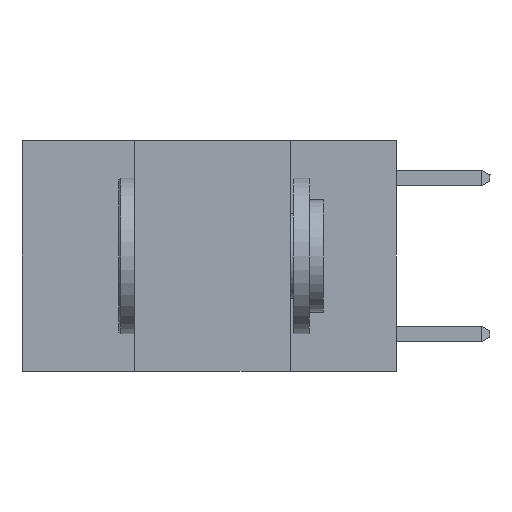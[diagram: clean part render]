
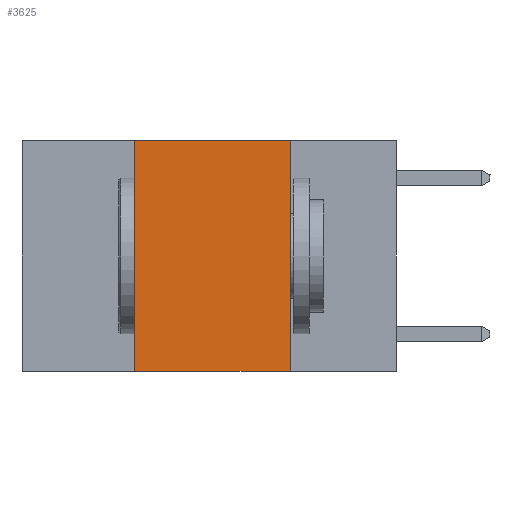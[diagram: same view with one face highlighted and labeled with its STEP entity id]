
A CAD part, left-side view. The second image highlights one B-rep face of the part: STEP entity #3625.
In plain terms, the highlighted planar face has unit normal (-1, 0, 0).
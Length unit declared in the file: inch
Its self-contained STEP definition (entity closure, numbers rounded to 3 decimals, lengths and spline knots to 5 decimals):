
#289 = CARTESIAN_POINT ( 'NONE',  ( 0., 0.6, 0. ) ) ;
#304 = PLANE ( 'NONE',  #2674 ) ;
#496 = VERTEX_POINT ( 'NONE', #10698 ) ;
#770 = CARTESIAN_POINT ( 'NONE',  ( 0., 0.42, -0.37 ) ) ;
#775 = VECTOR ( 'NONE', #3494, 39.37008 ) ;
#1143 = CARTESIAN_POINT ( 'NONE',  ( 0., 0.6, 0. ) ) ;
#1701 = LINE ( 'NONE', #289, #10487 ) ;
#1802 = CARTESIAN_POINT ( 'NONE',  ( 0., 0.42, 0. ) ) ;
#1816 = ORIENTED_EDGE ( 'NONE', *, *, #7473, .F. ) ;
#2242 = VERTEX_POINT ( 'NONE', #7618 ) ;
#2674 = AXIS2_PLACEMENT_3D ( 'NONE', #1143, #3521, #3466 ) ;
#3134 = CARTESIAN_POINT ( 'NONE',  ( 0., 0.17, 0. ) ) ;
#3329 = LINE ( 'NONE', #6118, #775 ) ;
#3409 = EDGE_CURVE ( 'NONE', #2242, #4586, #1701, .T. ) ;
#3466 = DIRECTION ( 'NONE',  ( 0., 0., -1. ) ) ;
#3494 = DIRECTION ( 'NONE',  ( 0., -1., 0. ) ) ;
#3521 = DIRECTION ( 'NONE',  ( 1., 0., 0. ) ) ;
#3625 = ADVANCED_FACE ( 'NONE', ( #8409 ), #304, .F. ) ;
#4297 = EDGE_CURVE ( 'NONE', #6660, #2242, #5740, .T. ) ;
#4416 = CARTESIAN_POINT ( 'NONE',  ( 0., 0.17, 0. ) ) ;
#4586 = VERTEX_POINT ( 'NONE', #3134 ) ;
#5119 = EDGE_LOOP ( 'NONE', ( #1816, #9589, #5320, #10456 ) ) ;
#5320 = ORIENTED_EDGE ( 'NONE', *, *, #4297, .F. ) ;
#5473 = VECTOR ( 'NONE', #8688, 39.37008 ) ;
#5740 = LINE ( 'NONE', #1802, #5473 ) ;
#6093 = LINE ( 'NONE', #4416, #6876 ) ;
#6118 = CARTESIAN_POINT ( 'NONE',  ( 0., 0.6, -0.37 ) ) ;
#6660 = VERTEX_POINT ( 'NONE', #770 ) ;
#6876 = VECTOR ( 'NONE', #10345, 39.37008 ) ;
#7473 = EDGE_CURVE ( 'NONE', #4586, #496, #6093, .T. ) ;
#7618 = CARTESIAN_POINT ( 'NONE',  ( 0., 0.42, 0. ) ) ;
#8409 = FACE_OUTER_BOUND ( 'NONE', #5119, .T. ) ;
#8652 = DIRECTION ( 'NONE',  ( 0., -1., 0. ) ) ;
#8688 = DIRECTION ( 'NONE',  ( 0., 0., 1. ) ) ;
#9099 = EDGE_CURVE ( 'NONE', #6660, #496, #3329, .T. ) ;
#9589 = ORIENTED_EDGE ( 'NONE', *, *, #3409, .F. ) ;
#10345 = DIRECTION ( 'NONE',  ( 0., 0., -1. ) ) ;
#10456 = ORIENTED_EDGE ( 'NONE', *, *, #9099, .T. ) ;
#10487 = VECTOR ( 'NONE', #8652, 39.37008 ) ;
#10698 = CARTESIAN_POINT ( 'NONE',  ( 0., 0.17, -0.37 ) ) ;
